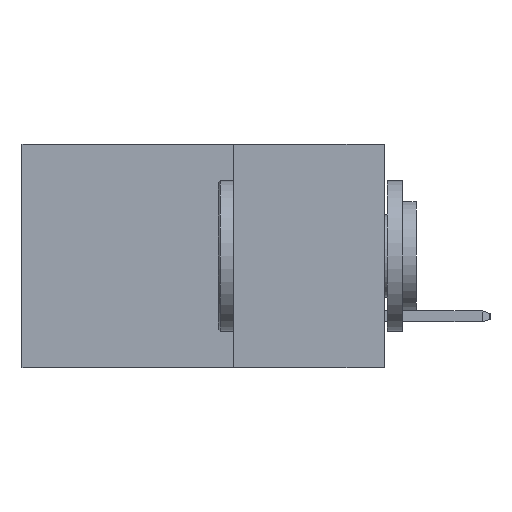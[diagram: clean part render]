
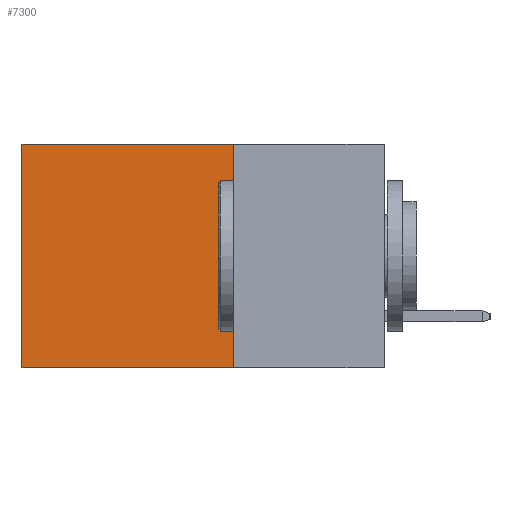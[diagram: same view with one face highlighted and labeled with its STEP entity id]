
A CAD part, left-side view. The second image highlights one B-rep face of the part: STEP entity #7300.
In plain terms, the highlighted planar face has unit normal (-1, 0, 0).
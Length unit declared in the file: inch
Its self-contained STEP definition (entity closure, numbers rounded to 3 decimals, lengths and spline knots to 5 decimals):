
#477 = CARTESIAN_POINT ( 'NONE',  ( 0.298, 0.25, -0.37 ) ) ;
#947 = DIRECTION ( 'NONE',  ( 0., 0., -1. ) ) ;
#1060 = VECTOR ( 'NONE', #8567, 39.37008 ) ;
#1391 = DIRECTION ( 'NONE',  ( 0., 0., -1. ) ) ;
#1609 = LINE ( 'NONE', #11458, #6657 ) ;
#3295 = EDGE_LOOP ( 'NONE', ( #8373, #8413, #8423, #8436 ) ) ;
#3385 = VERTEX_POINT ( 'NONE', #7056 ) ;
#3691 = CARTESIAN_POINT ( 'NONE',  ( 0.298, 0.25, -0.37 ) ) ;
#4407 = VERTEX_POINT ( 'NONE', #10369 ) ;
#5069 = VECTOR ( 'NONE', #9809, 39.37008 ) ;
#5141 = CARTESIAN_POINT ( 'NONE',  ( 0.298, 0.25, 0. ) ) ;
#5736 = DIRECTION ( 'NONE',  ( 0., 1., 0. ) ) ;
#6115 = DIRECTION ( 'NONE',  ( 1., 0., 0. ) ) ;
#6469 = LINE ( 'NONE', #3691, #1060 ) ;
#6483 = CARTESIAN_POINT ( 'NONE',  ( 0.298, 0.25, 0. ) ) ;
#6545 = VERTEX_POINT ( 'NONE', #6483 ) ;
#6657 = VECTOR ( 'NONE', #947, 39.37008 ) ;
#7056 = CARTESIAN_POINT ( 'NONE',  ( 0.298, 0.6, -0.37 ) ) ;
#7064 = VERTEX_POINT ( 'NONE', #477 ) ;
#7262 = EDGE_CURVE ( 'NONE', #4407, #3385, #1609, .T. ) ;
#7300 = ADVANCED_FACE ( 'NONE', ( #8587 ), #8935, .F. ) ;
#8225 = AXIS2_PLACEMENT_3D ( 'NONE', #11517, #6115, #1391 ) ;
#8373 = ORIENTED_EDGE ( 'NONE', *, *, #7262, .T. ) ;
#8413 = ORIENTED_EDGE ( 'NONE', *, *, #8880, .F. ) ;
#8423 = ORIENTED_EDGE ( 'NONE', *, *, #9186, .F. ) ;
#8436 = ORIENTED_EDGE ( 'NONE', *, *, #9627, .T. ) ;
#8567 = DIRECTION ( 'NONE',  ( 0., 1., 0. ) ) ;
#8587 = FACE_OUTER_BOUND ( 'NONE', #3295, .T. ) ;
#8880 = EDGE_CURVE ( 'NONE', #7064, #3385, #6469, .T. ) ;
#8935 = PLANE ( 'NONE',  #8225 ) ;
#9186 = EDGE_CURVE ( 'NONE', #6545, #7064, #12275, .T. ) ;
#9464 = CARTESIAN_POINT ( 'NONE',  ( 0.298, 0.25, 0. ) ) ;
#9627 = EDGE_CURVE ( 'NONE', #6545, #4407, #12266, .T. ) ;
#9809 = DIRECTION ( 'NONE',  ( 0., 0., -1. ) ) ;
#10011 = VECTOR ( 'NONE', #5736, 39.37008 ) ;
#10369 = CARTESIAN_POINT ( 'NONE',  ( 0.298, 0.6, 0. ) ) ;
#11458 = CARTESIAN_POINT ( 'NONE',  ( 0.298, 0.6, 0. ) ) ;
#11517 = CARTESIAN_POINT ( 'NONE',  ( 0.298, 0.25, 0. ) ) ;
#12266 = LINE ( 'NONE', #9464, #10011 ) ;
#12275 = LINE ( 'NONE', #5141, #5069 ) ;
